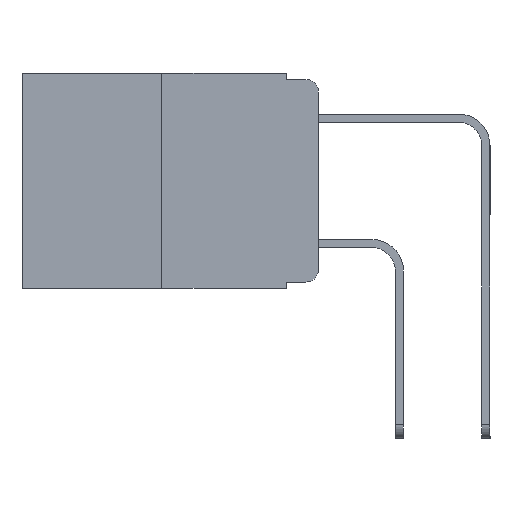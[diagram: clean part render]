
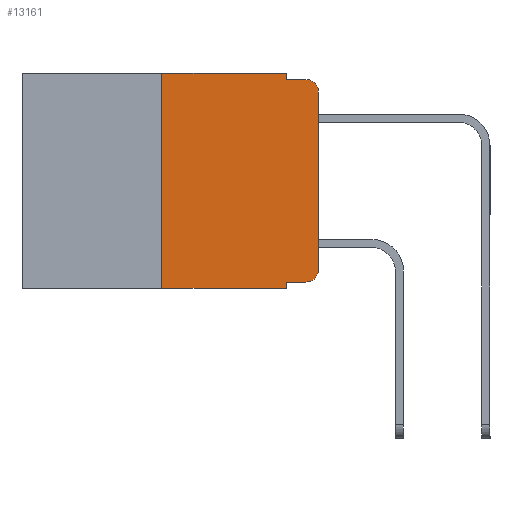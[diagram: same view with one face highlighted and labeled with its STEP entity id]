
A CAD part, left-side view. The second image highlights one B-rep face of the part: STEP entity #13161.
In plain terms, the highlighted planar face has unit normal (-1, 0, 0).
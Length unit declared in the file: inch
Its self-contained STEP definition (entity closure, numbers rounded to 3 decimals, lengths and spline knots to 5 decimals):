
#103 = DIRECTION ( 'NONE',  ( 0., 0., -1. ) ) ;
#114 = ORIENTED_EDGE ( 'NONE', *, *, #9322, .T. ) ;
#176 = CARTESIAN_POINT ( 'NONE',  ( 0., 0., 0. ) ) ;
#259 = CARTESIAN_POINT ( 'NONE',  ( 0., 0.051, 0. ) ) ;
#741 = EDGE_CURVE ( 'NONE', #9980, #5177, #7808, .T. ) ;
#852 = ORIENTED_EDGE ( 'NONE', *, *, #11444, .T. ) ;
#919 = LINE ( 'NONE', #11183, #3909 ) ;
#1002 = ORIENTED_EDGE ( 'NONE', *, *, #8471, .F. ) ;
#1074 = CARTESIAN_POINT ( 'NONE',  ( 0., 0., -0.313 ) ) ;
#1302 = VECTOR ( 'NONE', #2359, 39.37008 ) ;
#1564 = CARTESIAN_POINT ( 'NONE',  ( 0., 0.051, -0.333 ) ) ;
#1582 = DIRECTION ( 'NONE',  ( 0., -1., 0. ) ) ;
#1676 = LINE ( 'NONE', #7963, #1302 ) ;
#1712 = ORIENTED_EDGE ( 'NONE', *, *, #13750, .F. ) ;
#2039 = AXIS2_PLACEMENT_3D ( 'NONE', #5132, #12960, #6275 ) ;
#2061 = CARTESIAN_POINT ( 'NONE',  ( 0., 0.25, 0. ) ) ;
#2273 = CARTESIAN_POINT ( 'NONE',  ( 0., 0.473, 0. ) ) ;
#2359 = DIRECTION ( 'NONE',  ( 0., 0., -1. ) ) ;
#2515 = DIRECTION ( 'NONE',  ( 0., 0., -1. ) ) ;
#2776 = DIRECTION ( 'NONE',  ( 0., 0., -1. ) ) ;
#2777 = LINE ( 'NONE', #176, #8396 ) ;
#2810 = VECTOR ( 'NONE', #5431, 39.37008 ) ;
#3023 = VECTOR ( 'NONE', #12761, 39.37008 ) ;
#3075 = DIRECTION ( 'NONE',  ( -1., 0., 0. ) ) ;
#3091 = EDGE_CURVE ( 'NONE', #6751, #6348, #5996, .T. ) ;
#3581 = DIRECTION ( 'NONE',  ( 0., 0., 1. ) ) ;
#3909 = VECTOR ( 'NONE', #7743, 39.37008 ) ;
#3913 = CARTESIAN_POINT ( 'NONE',  ( 0., 0.02, -0.333 ) ) ;
#3992 = CARTESIAN_POINT ( 'NONE',  ( 0., 0.051, -0.01 ) ) ;
#4003 = VERTEX_POINT ( 'NONE', #3992 ) ;
#4492 = ORIENTED_EDGE ( 'NONE', *, *, #12938, .F. ) ;
#4511 = VECTOR ( 'NONE', #103, 39.37008 ) ;
#4665 = ORIENTED_EDGE ( 'NONE', *, *, #5326, .T. ) ;
#4684 = CARTESIAN_POINT ( 'NONE',  ( 0., 0.25, -0.343 ) ) ;
#4786 = ORIENTED_EDGE ( 'NONE', *, *, #3091, .T. ) ;
#4794 = VECTOR ( 'NONE', #1582, 39.37008 ) ;
#5102 = CARTESIAN_POINT ( 'NONE',  ( 0., 0.25, 0. ) ) ;
#5132 = CARTESIAN_POINT ( 'NONE',  ( 0., 0.02, -0.313 ) ) ;
#5177 = VERTEX_POINT ( 'NONE', #259 ) ;
#5279 = CIRCLE ( 'NONE', #2039, 0.02 ) ;
#5326 = EDGE_CURVE ( 'NONE', #11841, #8918, #13105, .T. ) ;
#5431 = DIRECTION ( 'NONE',  ( 0., 0., 1. ) ) ;
#5781 = CARTESIAN_POINT ( 'NONE',  ( 0., 0.473, 0. ) ) ;
#5996 = CIRCLE ( 'NONE', #12824, 0.02 ) ;
#6066 = CARTESIAN_POINT ( 'NONE',  ( 0., 0.02, -0.03 ) ) ;
#6275 = DIRECTION ( 'NONE',  ( 0., 0., -1. ) ) ;
#6348 = VERTEX_POINT ( 'NONE', #9042 ) ;
#6395 = EDGE_CURVE ( 'NONE', #10306, #6751, #2777, .T. ) ;
#6745 = ORIENTED_EDGE ( 'NONE', *, *, #6395, .T. ) ;
#6751 = VERTEX_POINT ( 'NONE', #11958 ) ;
#7205 = VECTOR ( 'NONE', #10855, 39.37008 ) ;
#7743 = DIRECTION ( 'NONE',  ( 0., -1., 0. ) ) ;
#7808 = LINE ( 'NONE', #2273, #4794 ) ;
#7907 = AXIS2_PLACEMENT_3D ( 'NONE', #5781, #9245, #2515 ) ;
#7963 = CARTESIAN_POINT ( 'NONE',  ( 0., 0.051, 0. ) ) ;
#8265 = EDGE_LOOP ( 'NONE', ( #6745, #4786, #11913, #1002, #12828, #4492, #4665, #1712, #114, #852 ) ) ;
#8396 = VECTOR ( 'NONE', #3581, 39.37008 ) ;
#8471 = EDGE_CURVE ( 'NONE', #5177, #4003, #1676, .T. ) ;
#8687 = VERTEX_POINT ( 'NONE', #3913 ) ;
#8918 = VERTEX_POINT ( 'NONE', #13185 ) ;
#9024 = EDGE_CURVE ( 'NONE', #4003, #6348, #919, .T. ) ;
#9042 = CARTESIAN_POINT ( 'NONE',  ( 0., 0.02, -0.01 ) ) ;
#9192 = PLANE ( 'NONE',  #7907 ) ;
#9245 = DIRECTION ( 'NONE',  ( 1., 0., 0. ) ) ;
#9295 = CARTESIAN_POINT ( 'NONE',  ( 0., 0.051, -0.333 ) ) ;
#9322 = EDGE_CURVE ( 'NONE', #11252, #8687, #9383, .T. ) ;
#9383 = LINE ( 'NONE', #1564, #3023 ) ;
#9980 = VERTEX_POINT ( 'NONE', #5102 ) ;
#10306 = VERTEX_POINT ( 'NONE', #1074 ) ;
#10528 = LINE ( 'NONE', #12425, #4511 ) ;
#10855 = DIRECTION ( 'NONE',  ( 0., -1., 0. ) ) ;
#11183 = CARTESIAN_POINT ( 'NONE',  ( 0., 0.051, -0.01 ) ) ;
#11252 = VERTEX_POINT ( 'NONE', #9295 ) ;
#11444 = EDGE_CURVE ( 'NONE', #8687, #10306, #5279, .T. ) ;
#11572 = FACE_OUTER_BOUND ( 'NONE', #8265, .T. ) ;
#11841 = VERTEX_POINT ( 'NONE', #4684 ) ;
#11898 = CARTESIAN_POINT ( 'NONE',  ( 0., 0.473, -0.343 ) ) ;
#11913 = ORIENTED_EDGE ( 'NONE', *, *, #9024, .F. ) ;
#11958 = CARTESIAN_POINT ( 'NONE',  ( 0., 0., -0.03 ) ) ;
#12078 = LINE ( 'NONE', #2061, #2810 ) ;
#12425 = CARTESIAN_POINT ( 'NONE',  ( 0., 0.051, 0. ) ) ;
#12761 = DIRECTION ( 'NONE',  ( 0., -1., 0. ) ) ;
#12824 = AXIS2_PLACEMENT_3D ( 'NONE', #6066, #3075, #2776 ) ;
#12828 = ORIENTED_EDGE ( 'NONE', *, *, #741, .F. ) ;
#12938 = EDGE_CURVE ( 'NONE', #11841, #9980, #12078, .T. ) ;
#12960 = DIRECTION ( 'NONE',  ( -1., 0., 0. ) ) ;
#13105 = LINE ( 'NONE', #11898, #7205 ) ;
#13161 = ADVANCED_FACE ( 'NONE', ( #11572 ), #9192, .F. ) ;
#13185 = CARTESIAN_POINT ( 'NONE',  ( 0., 0.051, -0.343 ) ) ;
#13750 = EDGE_CURVE ( 'NONE', #11252, #8918, #10528, .T. ) ;
